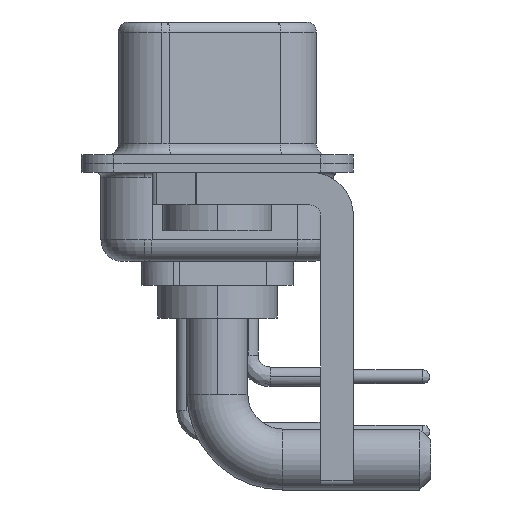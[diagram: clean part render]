
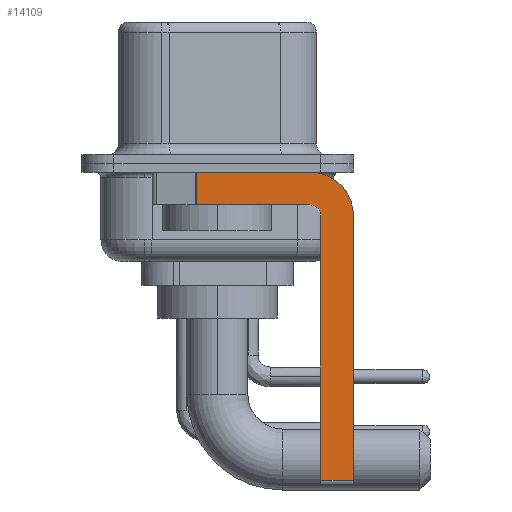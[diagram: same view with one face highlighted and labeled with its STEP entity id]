
A CAD part, left-side view. The second image highlights one B-rep face of the part: STEP entity #14109.
In plain terms, the highlighted planar face has unit normal (-1, 0, 0).
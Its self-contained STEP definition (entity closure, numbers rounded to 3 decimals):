
#308 = VECTOR ( 'NONE', #12199, 1000. ) ;
#757 = CARTESIAN_POINT ( 'NONE',  ( -2.9, -4.25, -0.4 ) ) ;
#1023 = CARTESIAN_POINT ( 'NONE',  ( -2.9, 0.978, -1.9 ) ) ;
#1159 = CARTESIAN_POINT ( 'NONE',  ( -2.9, -4.25, -2.4 ) ) ;
#1301 = VERTEX_POINT ( 'NONE', #757 ) ;
#1963 = AXIS2_PLACEMENT_3D ( 'NONE', #10500, #10647, #4855 ) ;
#2963 = VERTEX_POINT ( 'NONE', #18359 ) ;
#3001 = ORIENTED_EDGE ( 'NONE', *, *, #16233, .T. ) ;
#3725 = CARTESIAN_POINT ( 'NONE',  ( -2.9, -6.25, -2.4 ) ) ;
#3816 = VERTEX_POINT ( 'NONE', #3725 ) ;
#4578 = CARTESIAN_POINT ( 'NONE',  ( -2.9, 0.978, -1.9 ) ) ;
#4763 = CARTESIAN_POINT ( 'NONE',  ( -2.9, 0.978, -0.4 ) ) ;
#4828 = DIRECTION ( 'NONE',  ( 0., 0., -1. ) ) ;
#4855 = DIRECTION ( 'NONE',  ( 0., 0., 1. ) ) ;
#4951 = DIRECTION ( 'NONE',  ( 0., 0., -1. ) ) ;
#5596 = LINE ( 'NONE', #1023, #6526 ) ;
#5882 = CIRCLE ( 'NONE', #11032, 2. ) ;
#6526 = VECTOR ( 'NONE', #25493, 1000. ) ;
#6917 = CARTESIAN_POINT ( 'NONE',  ( -2.9, -4.25, -2.4 ) ) ;
#7112 = ORIENTED_EDGE ( 'NONE', *, *, #25021, .F. ) ;
#7795 = VERTEX_POINT ( 'NONE', #10450 ) ;
#7860 = CARTESIAN_POINT ( 'NONE',  ( -2.9, -6.25, -14.55 ) ) ;
#8163 = ORIENTED_EDGE ( 'NONE', *, *, #20039, .F. ) ;
#8740 = VERTEX_POINT ( 'NONE', #4763 ) ;
#8792 = DIRECTION ( 'NONE',  ( 0., 0., -1. ) ) ;
#9079 = EDGE_LOOP ( 'NONE', ( #14965, #3001, #20868, #9885, #8163, #15818, #18662, #7112 ) ) ;
#9192 = DIRECTION ( 'NONE',  ( 1., 0., 0. ) ) ;
#9885 = ORIENTED_EDGE ( 'NONE', *, *, #24375, .F. ) ;
#10099 = EDGE_CURVE ( 'NONE', #8740, #1301, #24144, .T. ) ;
#10450 = CARTESIAN_POINT ( 'NONE',  ( -2.9, -4.75, -14.55 ) ) ;
#10495 = CARTESIAN_POINT ( 'NONE',  ( -2.9, -4.75, -2.4 ) ) ;
#10500 = CARTESIAN_POINT ( 'NONE',  ( -2.9, -4.25, -2.4 ) ) ;
#10570 = CARTESIAN_POINT ( 'NONE',  ( -2.9, -4.75, -14.8 ) ) ;
#10647 = DIRECTION ( 'NONE',  ( -1., 0., 0. ) ) ;
#10895 = CARTESIAN_POINT ( 'NONE',  ( -2.9, -4.25, -14.55 ) ) ;
#10995 = EDGE_CURVE ( 'NONE', #7795, #22427, #25386, .T. ) ;
#11032 = AXIS2_PLACEMENT_3D ( 'NONE', #1159, #15180, #4951 ) ;
#12199 = DIRECTION ( 'NONE',  ( 0., -1., 0. ) ) ;
#12591 = DIRECTION ( 'NONE',  ( 0., 0., 1. ) ) ;
#12639 = DIRECTION ( 'NONE',  ( 0., -1., 0. ) ) ;
#12789 = CIRCLE ( 'NONE', #1963, 0.5 ) ;
#13599 = VECTOR ( 'NONE', #22955, 1000. ) ;
#14109 = ADVANCED_FACE ( 'NONE', ( #15121 ), #14845, .F. ) ;
#14516 = VECTOR ( 'NONE', #4828, 1000. ) ;
#14845 = PLANE ( 'NONE',  #21914 ) ;
#14965 = ORIENTED_EDGE ( 'NONE', *, *, #10099, .F. ) ;
#15121 = FACE_OUTER_BOUND ( 'NONE', #9079, .T. ) ;
#15180 = DIRECTION ( 'NONE',  ( 1., 0., 0. ) ) ;
#15818 = ORIENTED_EDGE ( 'NONE', *, *, #10995, .T. ) ;
#16233 = EDGE_CURVE ( 'NONE', #8740, #23031, #5596, .T. ) ;
#16528 = CARTESIAN_POINT ( 'NONE',  ( -2.9, -4.25, -1.9 ) ) ;
#16671 = LINE ( 'NONE', #17055, #14516 ) ;
#17055 = CARTESIAN_POINT ( 'NONE',  ( -2.9, -6.25, -2.4 ) ) ;
#18359 = CARTESIAN_POINT ( 'NONE',  ( -2.9, -4.25, -1.9 ) ) ;
#18662 = ORIENTED_EDGE ( 'NONE', *, *, #26246, .F. ) ;
#20039 = EDGE_CURVE ( 'NONE', #7795, #20878, #22785, .T. ) ;
#20384 = VECTOR ( 'NONE', #12591, 1000. ) ;
#20868 = ORIENTED_EDGE ( 'NONE', *, *, #24832, .F. ) ;
#20878 = VERTEX_POINT ( 'NONE', #10495 ) ;
#21914 = AXIS2_PLACEMENT_3D ( 'NONE', #6917, #9192, #8792 ) ;
#22398 = CARTESIAN_POINT ( 'NONE',  ( -2.9, 3., -0.4 ) ) ;
#22427 = VERTEX_POINT ( 'NONE', #7860 ) ;
#22785 = LINE ( 'NONE', #10570, #20384 ) ;
#22828 = LINE ( 'NONE', #16528, #13599 ) ;
#22955 = DIRECTION ( 'NONE',  ( 0., 1., 0. ) ) ;
#23031 = VERTEX_POINT ( 'NONE', #4578 ) ;
#24144 = LINE ( 'NONE', #22398, #308 ) ;
#24375 = EDGE_CURVE ( 'NONE', #20878, #2963, #12789, .T. ) ;
#24813 = VECTOR ( 'NONE', #12639, 1000. ) ;
#24832 = EDGE_CURVE ( 'NONE', #2963, #23031, #22828, .T. ) ;
#25021 = EDGE_CURVE ( 'NONE', #1301, #3816, #5882, .T. ) ;
#25386 = LINE ( 'NONE', #10895, #24813 ) ;
#25493 = DIRECTION ( 'NONE',  ( 0., 0., -1. ) ) ;
#26246 = EDGE_CURVE ( 'NONE', #3816, #22427, #16671, .T. ) ;
